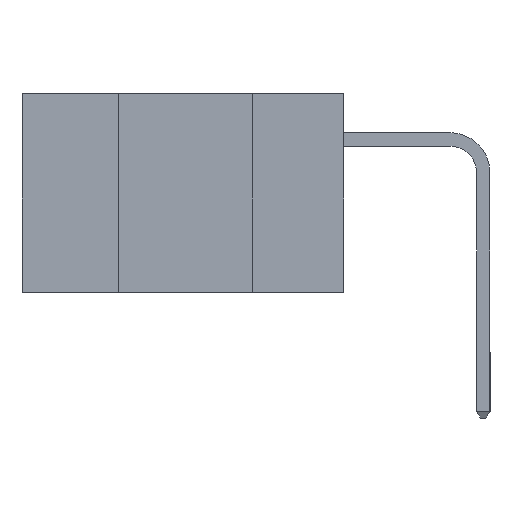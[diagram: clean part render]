
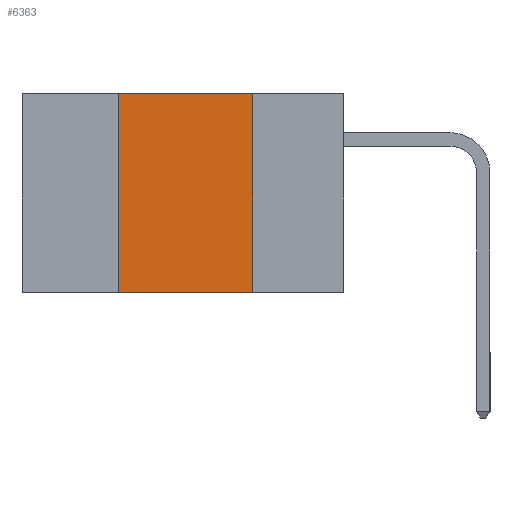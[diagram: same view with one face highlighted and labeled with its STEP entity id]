
A CAD part, left-side view. The second image highlights one B-rep face of the part: STEP entity #6363.
In plain terms, the highlighted planar face has unit normal (-1, 0, 0).
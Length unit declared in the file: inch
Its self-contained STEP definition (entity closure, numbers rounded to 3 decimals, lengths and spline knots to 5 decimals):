
#961 = LINE ( 'NONE', #8059, #5592 ) ;
#990 = ORIENTED_EDGE ( 'NONE', *, *, #10065, .F. ) ;
#1339 = CARTESIAN_POINT ( 'NONE',  ( 0., 0.17, 0. ) ) ;
#1971 = DIRECTION ( 'NONE',  ( 0., 0., -1. ) ) ;
#2006 = VERTEX_POINT ( 'NONE', #2203 ) ;
#2133 = VECTOR ( 'NONE', #1971, 39.37008 ) ;
#2182 = EDGE_LOOP ( 'NONE', ( #7923, #990, #2793, #2973 ) ) ;
#2203 = CARTESIAN_POINT ( 'NONE',  ( 0., 0.17, 0. ) ) ;
#2775 = CARTESIAN_POINT ( 'NONE',  ( 0., 0.17, -0.37 ) ) ;
#2793 = ORIENTED_EDGE ( 'NONE', *, *, #7072, .F. ) ;
#2973 = ORIENTED_EDGE ( 'NONE', *, *, #3653, .T. ) ;
#3114 = DIRECTION ( 'NONE',  ( 0., -1., 0. ) ) ;
#3653 = EDGE_CURVE ( 'NONE', #10348, #7579, #5856, .T. ) ;
#3973 = DIRECTION ( 'NONE',  ( 0., 0., 1. ) ) ;
#3976 = CARTESIAN_POINT ( 'NONE',  ( 0., 0.6, -0.37 ) ) ;
#4081 = CARTESIAN_POINT ( 'NONE',  ( 0., 0.42, 0. ) ) ;
#4209 = VECTOR ( 'NONE', #9695, 39.37008 ) ;
#4221 = CARTESIAN_POINT ( 'NONE',  ( 0., 0.6, 0. ) ) ;
#4796 = EDGE_CURVE ( 'NONE', #2006, #7579, #8868, .T. ) ;
#5592 = VECTOR ( 'NONE', #3973, 39.37008 ) ;
#5856 = LINE ( 'NONE', #3976, #9696 ) ;
#6363 = ADVANCED_FACE ( 'NONE', ( #9328 ), #7823, .F. ) ;
#6653 = VERTEX_POINT ( 'NONE', #4081 ) ;
#7072 = EDGE_CURVE ( 'NONE', #10348, #6653, #961, .T. ) ;
#7579 = VERTEX_POINT ( 'NONE', #2775 ) ;
#7690 = CARTESIAN_POINT ( 'NONE',  ( 0., 0.42, -0.37 ) ) ;
#7822 = CARTESIAN_POINT ( 'NONE',  ( 0., 0.6, 0. ) ) ;
#7823 = PLANE ( 'NONE',  #8410 ) ;
#7923 = ORIENTED_EDGE ( 'NONE', *, *, #4796, .F. ) ;
#8059 = CARTESIAN_POINT ( 'NONE',  ( 0., 0.42, 0. ) ) ;
#8410 = AXIS2_PLACEMENT_3D ( 'NONE', #7822, #10027, #10014 ) ;
#8868 = LINE ( 'NONE', #1339, #2133 ) ;
#9328 = FACE_OUTER_BOUND ( 'NONE', #2182, .T. ) ;
#9695 = DIRECTION ( 'NONE',  ( 0., -1., 0. ) ) ;
#9696 = VECTOR ( 'NONE', #3114, 39.37008 ) ;
#10014 = DIRECTION ( 'NONE',  ( 0., 0., -1. ) ) ;
#10027 = DIRECTION ( 'NONE',  ( 1., 0., 0. ) ) ;
#10065 = EDGE_CURVE ( 'NONE', #6653, #2006, #10416, .T. ) ;
#10348 = VERTEX_POINT ( 'NONE', #7690 ) ;
#10416 = LINE ( 'NONE', #4221, #4209 ) ;
